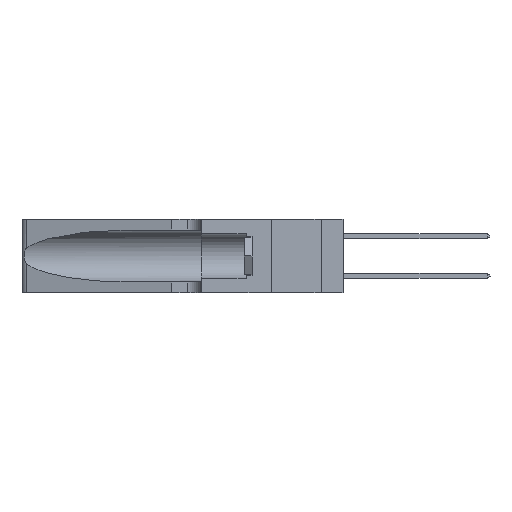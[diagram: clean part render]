
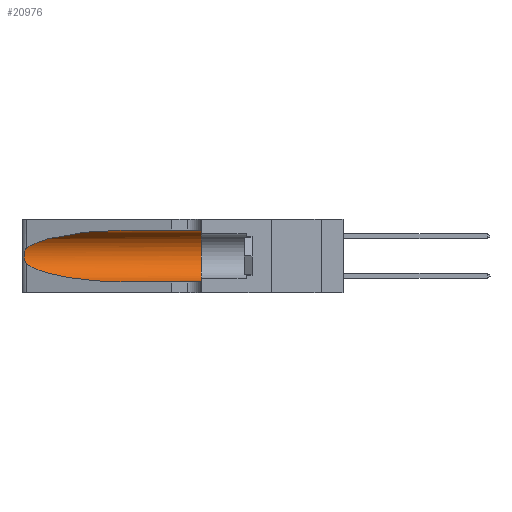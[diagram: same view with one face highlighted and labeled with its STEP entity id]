
A CAD part, left-side view. The second image highlights one B-rep face of the part: STEP entity #20976.
In plain terms, the highlighted cylindrical face has radius 3.308 mm (diameter 6.617 mm), a partial arc.
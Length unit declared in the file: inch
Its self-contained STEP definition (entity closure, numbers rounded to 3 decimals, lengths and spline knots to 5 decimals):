
#1064 = CARTESIAN_POINT ( 'NONE',  ( 0.1305, 1.61858, 0.185 ) ) ;
#1248 = AXIS2_PLACEMENT_3D ( 'NONE', #4241, #19999, #29691 ) ;
#1968 = CARTESIAN_POINT ( 'NONE',  ( 0.25787, 1.23484, 0.2124 ) ) ;
#2005 = CARTESIAN_POINT ( 'NONE',  ( 0.1305, 0.35, 0.31525 ) ) ;
#3084 = FACE_OUTER_BOUND ( 'NONE', #15935, .T. ) ;
#3841 = CARTESIAN_POINT ( 'NONE',  ( 0.25487, 1.22718, 0.14631 ) ) ;
#4241 = CARTESIAN_POINT ( 'NONE',  ( 0.1305, 0.35, 0.185 ) ) ;
#4455 = CARTESIAN_POINT ( 'NONE',  ( 0.25856, 1.23593, 0.16098 ) ) ;
#5289 = CARTESIAN_POINT ( 'NONE',  ( 0.25487, 1.22718, 0.14631 ) ) ;
#5425 = CARTESIAN_POINT ( 'NONE',  ( 0.25789, 1.23486, 0.15765 ) ) ;
#6398 = CIRCLE ( 'NONE', #1248, 0.13025 ) ;
#7526 = CARTESIAN_POINT ( 'NONE',  ( 0.26018, 1.23835, 0.19895 ) ) ;
#7744 = VECTOR ( 'NONE', #8195, 39.37008 ) ;
#8195 = DIRECTION ( 'NONE',  ( 0., -1., 0. ) ) ;
#8551 = VERTEX_POINT ( 'NONE', #2005 ) ;
#8754 = CARTESIAN_POINT ( 'NONE',  ( 0.18966, 0.96281, 0.05475 ) ) ;
#9183 = EDGE_CURVE ( 'NONE', #31541, #35811, #27017, .T. ) ;
#10369 = CARTESIAN_POINT ( 'NONE',  ( 0.2373, 1.15595, 0.28018 ) ) ;
#11404 = EDGE_CURVE ( 'NONE', #35811, #13693, #26153, .T. ) ;
#11884 = EDGE_CURVE ( 'NONE', #24742, #29771, #30830, .T. ) ;
#13186 = ORIENTED_EDGE ( 'NONE', *, *, #17284, .T. ) ;
#13693 = VERTEX_POINT ( 'NONE', #26787 ) ;
#13841 = CARTESIAN_POINT ( 'NONE',  ( 0.25639, 1.23186, 0.15144 ) ) ;
#14097 = CARTESIAN_POINT ( 'NONE',  ( 0.25854, 1.2359, 0.20912 ) ) ;
#15935 = EDGE_LOOP ( 'NONE', ( #26258, #13186, #29686, #22215, #26001, #25068 ) ) ;
#16583 = CYLINDRICAL_SURFACE ( 'NONE', #29547, 0.13025 ) ;
#16734 = CARTESIAN_POINT ( 'NONE',  ( 0.1305, 0.72297, 0.31525 ) ) ;
#17077 = DIRECTION ( 'NONE',  ( 0., -1., 0. ) ) ;
#17284 = EDGE_CURVE ( 'NONE', #29771, #31541, #32616, .T. ) ;
#17302 = CARTESIAN_POINT ( 'NONE',  ( 0.25555, 1.22994, 0.2215 ) ) ;
#17446 = CARTESIAN_POINT ( 'NONE',  ( 0.1305, 1.61858, 0.31525 ) ) ;
#18481 = CARTESIAN_POINT ( 'NONE',  ( 0.1305, 0.72297, 0.31525 ) ) ;
#19620 = CARTESIAN_POINT ( 'NONE',  ( 0.25487, 1.22718, 0.22369 ) ) ;
#19878 = VECTOR ( 'NONE', #30613, 39.37008 ) ;
#19999 = DIRECTION ( 'NONE',  ( 0., 1., 0. ) ) ;
#20504 = CARTESIAN_POINT ( 'NONE',  ( 0.26017, 1.23833, 0.17102 ) ) ;
#20976 = ADVANCED_FACE ( 'NONE', ( #3084 ), #16583, .F. ) ;
#22215 = ORIENTED_EDGE ( 'NONE', *, *, #11404, .T. ) ;
#23396 = CARTESIAN_POINT ( 'NONE',  ( 0.26075, 1.23896, 0.178 ) ) ;
#24336 = LINE ( 'NONE', #17446, #19878 ) ;
#24340 = CARTESIAN_POINT ( 'NONE',  ( 0.1305, 0.72297, 0.05475 ) ) ;
#24742 = VERTEX_POINT ( 'NONE', #18481 ) ;
#25068 = ORIENTED_EDGE ( 'NONE', *, *, #31149, .F. ) ;
#26001 = ORIENTED_EDGE ( 'NONE', *, *, #30348, .F. ) ;
#26153 = LINE ( 'NONE', #39713, #7744 ) ;
#26258 = ORIENTED_EDGE ( 'NONE', *, *, #11884, .T. ) ;
#26787 = CARTESIAN_POINT ( 'NONE',  ( 0.1305, 0.35, 0.05475 ) ) ;
#27017 =( BOUNDED_CURVE ( )  B_SPLINE_CURVE ( 3, ( #27753, #40652, #8754, #40125 ),
 .UNSPECIFIED., .F., .F. ) 
 B_SPLINE_CURVE_WITH_KNOTS ( ( 4, 4 ),
 ( 3.44316, 4.71239 ),
 .UNSPECIFIED. ) 
 CURVE ( )  GEOMETRIC_REPRESENTATION_ITEM ( )  RATIONAL_B_SPLINE_CURVE ( ( 1., 0.87, 0.87, 1. ) ) 
 REPRESENTATION_ITEM ( '' )  );
#27411 = CARTESIAN_POINT ( 'NONE',  ( 0.26075, 1.23896, 0.19203 ) ) ;
#27753 = CARTESIAN_POINT ( 'NONE',  ( 0.25487, 1.22718, 0.14631 ) ) ;
#29547 = AXIS2_PLACEMENT_3D ( 'NONE', #1064, #17077, #38971 ) ;
#29686 = ORIENTED_EDGE ( 'NONE', *, *, #9183, .T. ) ;
#29691 = DIRECTION ( 'NONE',  ( 0., 0., 1. ) ) ;
#29771 = VERTEX_POINT ( 'NONE', #19620 ) ;
#30348 = EDGE_CURVE ( 'NONE', #8551, #13693, #6398, .T. ) ;
#30613 = DIRECTION ( 'NONE',  ( 0., -1., 0. ) ) ;
#30830 =( BOUNDED_CURVE ( )  B_SPLINE_CURVE ( 3, ( #16734, #39044, #10369, #32819 ),
 .UNSPECIFIED., .F., .F. ) 
 B_SPLINE_CURVE_WITH_KNOTS ( ( 4, 4 ),
 ( 1.5708, 2.84003 ),
 .UNSPECIFIED. ) 
 CURVE ( )  GEOMETRIC_REPRESENTATION_ITEM ( )  RATIONAL_B_SPLINE_CURVE ( ( 1., 0.87, 0.87, 1. ) ) 
 REPRESENTATION_ITEM ( '' )  );
#31149 = EDGE_CURVE ( 'NONE', #24742, #8551, #24336, .T. ) ;
#31541 = VERTEX_POINT ( 'NONE', #3841 ) ;
#32616 = B_SPLINE_CURVE_WITH_KNOTS ( 'NONE', 3,
 ( #37108, #17302, #33097, #1968, #14097, #7526, #27411, #23396, #20504, #4455, #5425, #13841, #35994, #5289 ),
 .UNSPECIFIED., .F., .F.,
 ( 4, 2, 2, 2, 2, 2, 4 ),
 ( 0., 0.00027, 0.00053, 0.00107, 0.0016, 0.00187, 0.00214 ),
 .UNSPECIFIED. ) ;
#32819 = CARTESIAN_POINT ( 'NONE',  ( 0.25487, 1.22718, 0.22369 ) ) ;
#33097 = CARTESIAN_POINT ( 'NONE',  ( 0.25639, 1.23184, 0.21858 ) ) ;
#35811 = VERTEX_POINT ( 'NONE', #24340 ) ;
#35994 = CARTESIAN_POINT ( 'NONE',  ( 0.25555, 1.22993, 0.14849 ) ) ;
#37108 = CARTESIAN_POINT ( 'NONE',  ( 0.25487, 1.22718, 0.22369 ) ) ;
#38971 = DIRECTION ( 'NONE',  ( 0., 0., -1. ) ) ;
#39044 = CARTESIAN_POINT ( 'NONE',  ( 0.18966, 0.96281, 0.31525 ) ) ;
#39713 = CARTESIAN_POINT ( 'NONE',  ( 0.1305, 1.61858, 0.05475 ) ) ;
#40125 = CARTESIAN_POINT ( 'NONE',  ( 0.1305, 0.72297, 0.05475 ) ) ;
#40652 = CARTESIAN_POINT ( 'NONE',  ( 0.2373, 1.15595, 0.08982 ) ) ;
